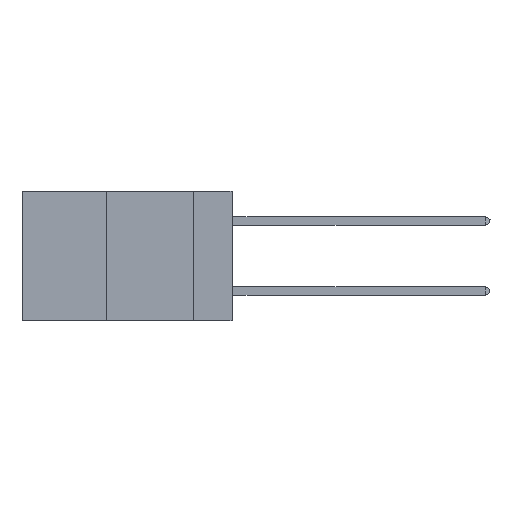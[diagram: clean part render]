
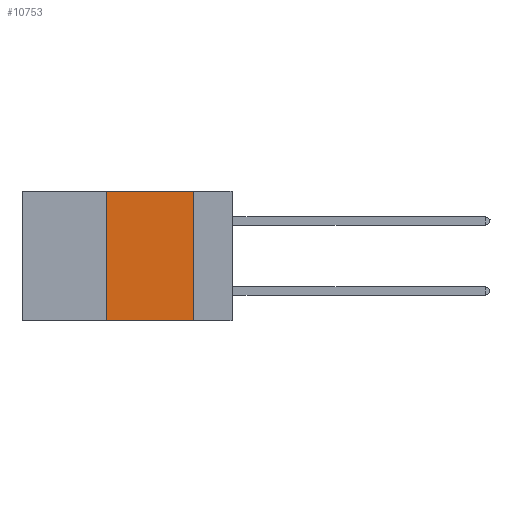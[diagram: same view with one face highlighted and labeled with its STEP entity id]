
A CAD part, left-side view. The second image highlights one B-rep face of the part: STEP entity #10753.
In plain terms, the highlighted planar face has unit normal (-1, 0, 0).
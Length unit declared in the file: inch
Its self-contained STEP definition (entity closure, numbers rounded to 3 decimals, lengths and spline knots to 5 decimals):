
#30 = VERTEX_POINT ( 'NONE', #5310 ) ;
#558 = ORIENTED_EDGE ( 'NONE', *, *, #10991, .T. ) ;
#628 = CARTESIAN_POINT ( 'NONE',  ( 0., 0.6, -0.37 ) ) ;
#795 = VERTEX_POINT ( 'NONE', #11305 ) ;
#1432 = VECTOR ( 'NONE', #8897, 39.37008 ) ;
#2391 = ORIENTED_EDGE ( 'NONE', *, *, #4643, .F. ) ;
#2492 = PLANE ( 'NONE',  #8841 ) ;
#2585 = FACE_OUTER_BOUND ( 'NONE', #12416, .T. ) ;
#3101 = LINE ( 'NONE', #6066, #7997 ) ;
#3106 = CARTESIAN_POINT ( 'NONE',  ( 0., 0.11, 0. ) ) ;
#4072 = CARTESIAN_POINT ( 'NONE',  ( 0., 0.11, -0.37 ) ) ;
#4401 = ORIENTED_EDGE ( 'NONE', *, *, #14405, .F. ) ;
#4643 = EDGE_CURVE ( 'NONE', #18184, #15081, #13294, .T. ) ;
#4882 = LINE ( 'NONE', #628, #1432 ) ;
#5310 = CARTESIAN_POINT ( 'NONE',  ( 0., 0.36, -0.37 ) ) ;
#6066 = CARTESIAN_POINT ( 'NONE',  ( 0., 0.6, 0. ) ) ;
#6301 = CARTESIAN_POINT ( 'NONE',  ( 0., 0.36, 0. ) ) ;
#6480 = VECTOR ( 'NONE', #12445, 39.37008 ) ;
#6524 = EDGE_CURVE ( 'NONE', #30, #795, #6577, .T. ) ;
#6577 = LINE ( 'NONE', #6301, #18226 ) ;
#6872 = CARTESIAN_POINT ( 'NONE',  ( 0., 0.11, 0. ) ) ;
#7997 = VECTOR ( 'NONE', #10447, 39.37008 ) ;
#8841 = AXIS2_PLACEMENT_3D ( 'NONE', #10854, #18137, #18221 ) ;
#8897 = DIRECTION ( 'NONE',  ( 0., -1., 0. ) ) ;
#9454 = ORIENTED_EDGE ( 'NONE', *, *, #6524, .F. ) ;
#10447 = DIRECTION ( 'NONE',  ( 0., -1., 0. ) ) ;
#10753 = ADVANCED_FACE ( 'NONE', ( #2585 ), #2492, .F. ) ;
#10854 = CARTESIAN_POINT ( 'NONE',  ( 0., 0.6, 0. ) ) ;
#10991 = EDGE_CURVE ( 'NONE', #30, #15081, #4882, .T. ) ;
#11305 = CARTESIAN_POINT ( 'NONE',  ( 0., 0.36, 0. ) ) ;
#12416 = EDGE_LOOP ( 'NONE', ( #2391, #4401, #9454, #558 ) ) ;
#12445 = DIRECTION ( 'NONE',  ( 0., 0., -1. ) ) ;
#13294 = LINE ( 'NONE', #6872, #6480 ) ;
#14405 = EDGE_CURVE ( 'NONE', #795, #18184, #3101, .T. ) ;
#15081 = VERTEX_POINT ( 'NONE', #4072 ) ;
#16428 = DIRECTION ( 'NONE',  ( 0., 0., 1. ) ) ;
#18137 = DIRECTION ( 'NONE',  ( 1., 0., 0. ) ) ;
#18184 = VERTEX_POINT ( 'NONE', #3106 ) ;
#18221 = DIRECTION ( 'NONE',  ( 0., 0., -1. ) ) ;
#18226 = VECTOR ( 'NONE', #16428, 39.37008 ) ;
